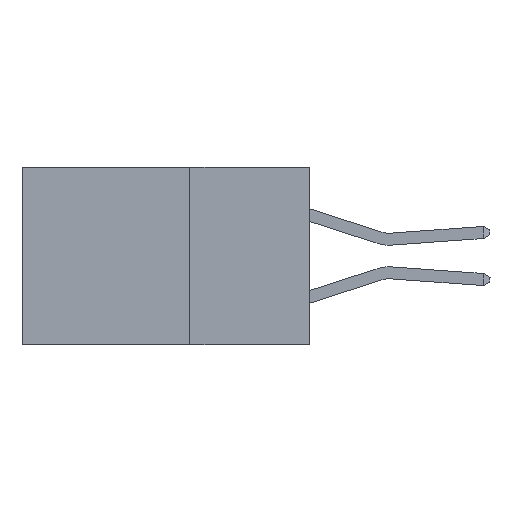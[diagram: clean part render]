
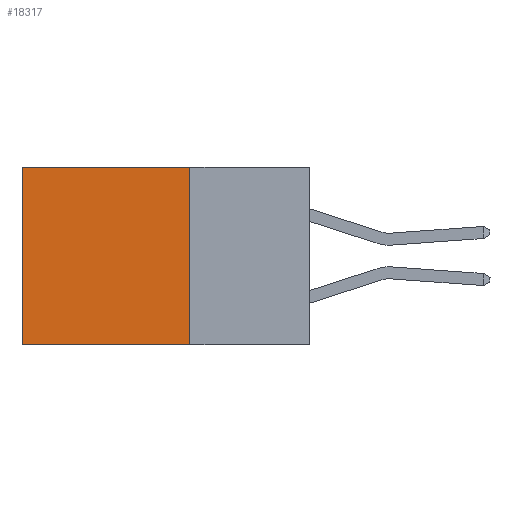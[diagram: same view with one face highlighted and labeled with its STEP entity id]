
A CAD part, left-side view. The second image highlights one B-rep face of the part: STEP entity #18317.
In plain terms, the highlighted planar face has unit normal (-1, 0, 0).
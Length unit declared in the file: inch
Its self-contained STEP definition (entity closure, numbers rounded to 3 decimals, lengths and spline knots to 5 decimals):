
#2063 = CARTESIAN_POINT ( 'NONE',  ( 0.298, 0.6, 0. ) ) ;
#2071 = DIRECTION ( 'NONE',  ( 0., 0., -1. ) ) ;
#3065 = CARTESIAN_POINT ( 'NONE',  ( 0.298, 0.25, 0. ) ) ;
#3354 = AXIS2_PLACEMENT_3D ( 'NONE', #20789, #19153, #20861 ) ;
#3947 = VECTOR ( 'NONE', #14397, 39.37008 ) ;
#4362 = DIRECTION ( 'NONE',  ( 0., 1., 0. ) ) ;
#4427 = ORIENTED_EDGE ( 'NONE', *, *, #8642, .T. ) ;
#4909 = VECTOR ( 'NONE', #4362, 39.37008 ) ;
#5121 = FACE_OUTER_BOUND ( 'NONE', #8942, .T. ) ;
#5239 = CARTESIAN_POINT ( 'NONE',  ( 0.298, 0.25, -0.37 ) ) ;
#5241 = ORIENTED_EDGE ( 'NONE', *, *, #16527, .T. ) ;
#5511 = EDGE_CURVE ( 'NONE', #16516, #19028, #14067, .T. ) ;
#6009 = LINE ( 'NONE', #7845, #4909 ) ;
#6806 = VECTOR ( 'NONE', #9977, 39.37008 ) ;
#6990 = CARTESIAN_POINT ( 'NONE',  ( 0.298, 0.6, -0.37 ) ) ;
#7845 = CARTESIAN_POINT ( 'NONE',  ( 0.298, 0.25, 0. ) ) ;
#8642 = EDGE_CURVE ( 'NONE', #16516, #17821, #6009, .T. ) ;
#8803 = ORIENTED_EDGE ( 'NONE', *, *, #5511, .F. ) ;
#8859 = PLANE ( 'NONE',  #3354 ) ;
#8942 = EDGE_LOOP ( 'NONE', ( #5241, #14802, #8803, #4427 ) ) ;
#9977 = DIRECTION ( 'NONE',  ( 0., 0., -1. ) ) ;
#10435 = VERTEX_POINT ( 'NONE', #6990 ) ;
#11444 = LINE ( 'NONE', #15102, #6806 ) ;
#12432 = CARTESIAN_POINT ( 'NONE',  ( 0.298, 0.25, 0. ) ) ;
#12664 = CARTESIAN_POINT ( 'NONE',  ( 0.298, 0.25, -0.37 ) ) ;
#14067 = LINE ( 'NONE', #12432, #15928 ) ;
#14397 = DIRECTION ( 'NONE',  ( 0., 1., 0. ) ) ;
#14802 = ORIENTED_EDGE ( 'NONE', *, *, #19513, .F. ) ;
#15102 = CARTESIAN_POINT ( 'NONE',  ( 0.298, 0.6, 0. ) ) ;
#15928 = VECTOR ( 'NONE', #2071, 39.37008 ) ;
#16516 = VERTEX_POINT ( 'NONE', #3065 ) ;
#16527 = EDGE_CURVE ( 'NONE', #17821, #10435, #11444, .T. ) ;
#17821 = VERTEX_POINT ( 'NONE', #2063 ) ;
#18317 = ADVANCED_FACE ( 'NONE', ( #5121 ), #8859, .F. ) ;
#19028 = VERTEX_POINT ( 'NONE', #5239 ) ;
#19153 = DIRECTION ( 'NONE',  ( 1., 0., 0. ) ) ;
#19317 = LINE ( 'NONE', #12664, #3947 ) ;
#19513 = EDGE_CURVE ( 'NONE', #19028, #10435, #19317, .T. ) ;
#20789 = CARTESIAN_POINT ( 'NONE',  ( 0.298, 0.25, 0. ) ) ;
#20861 = DIRECTION ( 'NONE',  ( 0., 0., -1. ) ) ;
